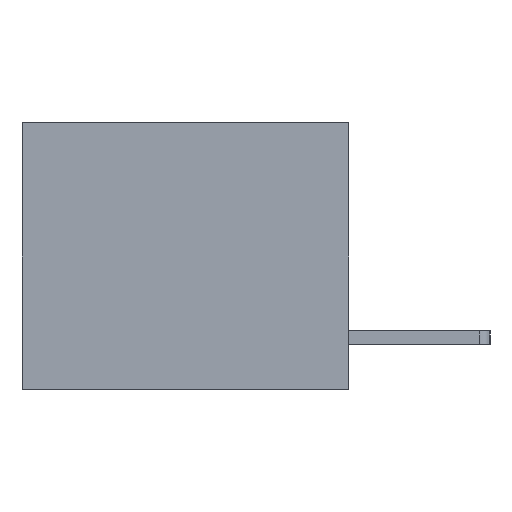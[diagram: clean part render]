
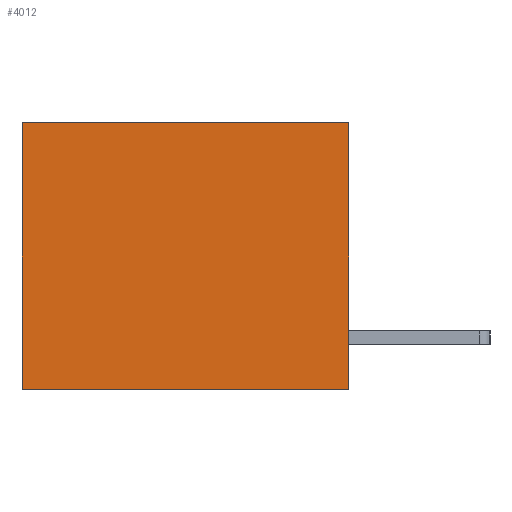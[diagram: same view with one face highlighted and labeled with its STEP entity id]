
A CAD part, left-side view. The second image highlights one B-rep face of the part: STEP entity #4012.
In plain terms, the highlighted planar face has unit normal (-1, 0, 0).
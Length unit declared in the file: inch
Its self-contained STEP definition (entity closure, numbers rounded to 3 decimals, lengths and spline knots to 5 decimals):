
#12 = CARTESIAN_POINT ( 'NONE',  ( 0.3165, 0., -0.49 ) ) ;
#314 = LINE ( 'NONE', #5798, #4290 ) ;
#438 = VERTEX_POINT ( 'NONE', #8121 ) ;
#629 = ORIENTED_EDGE ( 'NONE', *, *, #1573, .F. ) ;
#631 = LINE ( 'NONE', #10434, #2851 ) ;
#663 = DIRECTION ( 'NONE',  ( 0., 0., -1. ) ) ;
#936 = LINE ( 'NONE', #3534, #9736 ) ;
#1497 = EDGE_CURVE ( 'NONE', #8574, #438, #936, .T. ) ;
#1573 = EDGE_CURVE ( 'NONE', #4522, #6187, #631, .T. ) ;
#1728 = PLANE ( 'NONE',  #10420 ) ;
#2465 = CARTESIAN_POINT ( 'NONE',  ( 0.3165, 0., -0.49 ) ) ;
#2851 = VECTOR ( 'NONE', #9479, 39.37008 ) ;
#3046 = LINE ( 'NONE', #3522, #7817 ) ;
#3429 = DIRECTION ( 'NONE',  ( 0., 0., -1. ) ) ;
#3522 = CARTESIAN_POINT ( 'NONE',  ( 0.3165, 0., -0.49 ) ) ;
#3534 = CARTESIAN_POINT ( 'NONE',  ( 0.3165, 0., 0. ) ) ;
#4012 = ADVANCED_FACE ( 'NONE', ( #7336 ), #1728, .F. ) ;
#4290 = VECTOR ( 'NONE', #6154, 39.37008 ) ;
#4522 = VERTEX_POINT ( 'NONE', #12 ) ;
#5798 = CARTESIAN_POINT ( 'NONE',  ( 0.3165, 0.6, -0.49 ) ) ;
#6154 = DIRECTION ( 'NONE',  ( 0., 0., -1. ) ) ;
#6187 = VERTEX_POINT ( 'NONE', #10460 ) ;
#6307 = DIRECTION ( 'NONE',  ( 0., 1., 0. ) ) ;
#6431 = CARTESIAN_POINT ( 'NONE',  ( 0.3165, 0., 0. ) ) ;
#7336 = FACE_OUTER_BOUND ( 'NONE', #8157, .T. ) ;
#7435 = ORIENTED_EDGE ( 'NONE', *, *, #1497, .T. ) ;
#7676 = EDGE_CURVE ( 'NONE', #438, #6187, #314, .T. ) ;
#7817 = VECTOR ( 'NONE', #663, 39.37008 ) ;
#8044 = EDGE_CURVE ( 'NONE', #8574, #4522, #3046, .T. ) ;
#8121 = CARTESIAN_POINT ( 'NONE',  ( 0.3165, 0.6, 0. ) ) ;
#8157 = EDGE_LOOP ( 'NONE', ( #10755, #629, #8526, #7435 ) ) ;
#8526 = ORIENTED_EDGE ( 'NONE', *, *, #8044, .F. ) ;
#8574 = VERTEX_POINT ( 'NONE', #6431 ) ;
#9154 = DIRECTION ( 'NONE',  ( 1., 0., 0. ) ) ;
#9479 = DIRECTION ( 'NONE',  ( 0., 1., 0. ) ) ;
#9736 = VECTOR ( 'NONE', #6307, 39.37008 ) ;
#10420 = AXIS2_PLACEMENT_3D ( 'NONE', #2465, #9154, #3429 ) ;
#10434 = CARTESIAN_POINT ( 'NONE',  ( 0.3165, 0., -0.49 ) ) ;
#10460 = CARTESIAN_POINT ( 'NONE',  ( 0.3165, 0.6, -0.49 ) ) ;
#10755 = ORIENTED_EDGE ( 'NONE', *, *, #7676, .T. ) ;
